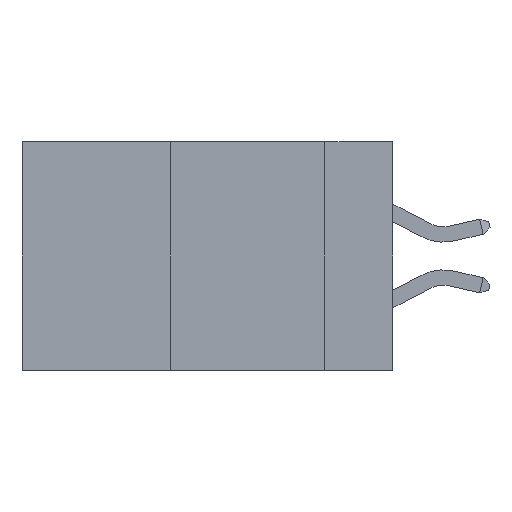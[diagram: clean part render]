
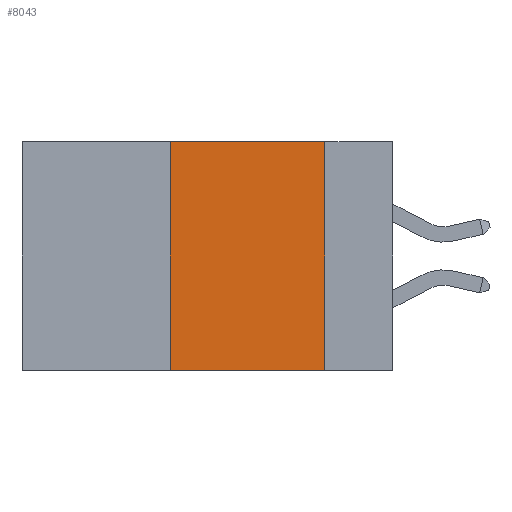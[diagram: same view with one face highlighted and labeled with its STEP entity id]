
A CAD part, left-side view. The second image highlights one B-rep face of the part: STEP entity #8043.
In plain terms, the highlighted planar face has unit normal (-1, 0, 0).
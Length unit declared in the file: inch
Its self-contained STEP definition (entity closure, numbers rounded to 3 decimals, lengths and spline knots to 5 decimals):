
#460 = EDGE_LOOP ( 'NONE', ( #5318, #9335, #1727, #11084 ) ) ;
#1198 = LINE ( 'NONE', #11742, #9552 ) ;
#1727 = ORIENTED_EDGE ( 'NONE', *, *, #13248, .F. ) ;
#1773 = CARTESIAN_POINT ( 'NONE',  ( 0., 0.6, 0. ) ) ;
#2244 = DIRECTION ( 'NONE',  ( 0., 0., -1. ) ) ;
#2633 = DIRECTION ( 'NONE',  ( 0., -1., 0. ) ) ;
#3036 = PLANE ( 'NONE',  #14851 ) ;
#3844 = VERTEX_POINT ( 'NONE', #5616 ) ;
#4026 = CARTESIAN_POINT ( 'NONE',  ( 0., 0.11, 0. ) ) ;
#4074 = EDGE_CURVE ( 'NONE', #7799, #6040, #8748, .T. ) ;
#4300 = FACE_OUTER_BOUND ( 'NONE', #460, .T. ) ;
#4368 = VECTOR ( 'NONE', #9706, 39.37008 ) ;
#4769 = CARTESIAN_POINT ( 'NONE',  ( 0., 0.11, -0.37 ) ) ;
#5066 = CARTESIAN_POINT ( 'NONE',  ( 0., 0.6, 0. ) ) ;
#5250 = EDGE_CURVE ( 'NONE', #6040, #9363, #1198, .T. ) ;
#5318 = ORIENTED_EDGE ( 'NONE', *, *, #5250, .F. ) ;
#5616 = CARTESIAN_POINT ( 'NONE',  ( 0., 0.36, -0.37 ) ) ;
#6040 = VERTEX_POINT ( 'NONE', #4026 ) ;
#7799 = VERTEX_POINT ( 'NONE', #11293 ) ;
#7806 = DIRECTION ( 'NONE',  ( 0., 0., -1. ) ) ;
#8043 = ADVANCED_FACE ( 'NONE', ( #4300 ), #3036, .F. ) ;
#8263 = VECTOR ( 'NONE', #2633, 39.37008 ) ;
#8748 = LINE ( 'NONE', #5066, #8263 ) ;
#8778 = LINE ( 'NONE', #14746, #9158 ) ;
#9158 = VECTOR ( 'NONE', #10026, 39.37008 ) ;
#9335 = ORIENTED_EDGE ( 'NONE', *, *, #4074, .F. ) ;
#9363 = VERTEX_POINT ( 'NONE', #4769 ) ;
#9481 = EDGE_CURVE ( 'NONE', #3844, #9363, #12136, .T. ) ;
#9552 = VECTOR ( 'NONE', #2244, 39.37008 ) ;
#9706 = DIRECTION ( 'NONE',  ( 0., -1., 0. ) ) ;
#10026 = DIRECTION ( 'NONE',  ( 0., 0., 1. ) ) ;
#11084 = ORIENTED_EDGE ( 'NONE', *, *, #9481, .T. ) ;
#11293 = CARTESIAN_POINT ( 'NONE',  ( 0., 0.36, 0. ) ) ;
#11742 = CARTESIAN_POINT ( 'NONE',  ( 0., 0.11, 0. ) ) ;
#12054 = CARTESIAN_POINT ( 'NONE',  ( 0., 0.6, -0.37 ) ) ;
#12136 = LINE ( 'NONE', #12054, #4368 ) ;
#13248 = EDGE_CURVE ( 'NONE', #3844, #7799, #8778, .T. ) ;
#14746 = CARTESIAN_POINT ( 'NONE',  ( 0., 0.36, 0. ) ) ;
#14851 = AXIS2_PLACEMENT_3D ( 'NONE', #1773, #14895, #7806 ) ;
#14895 = DIRECTION ( 'NONE',  ( 1., 0., 0. ) ) ;
